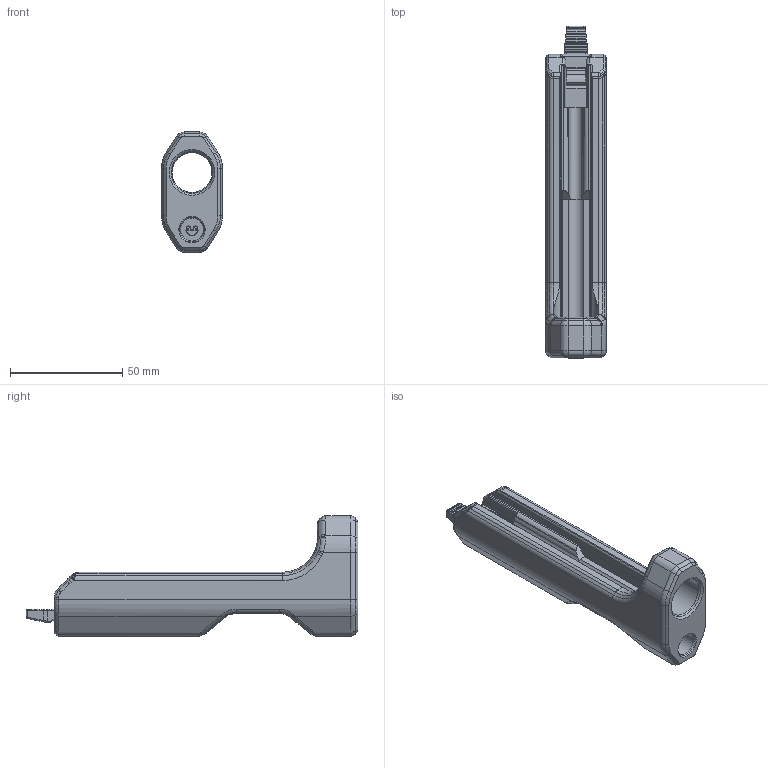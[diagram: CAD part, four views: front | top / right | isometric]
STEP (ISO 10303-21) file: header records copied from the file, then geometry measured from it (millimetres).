
FILE_DESCRIPTION(/* description */ (''),/* implementation_level */ '2;1');
FILE_NAME(/* name */ '10mm Spike Mount.step',/* time_stamp */ '2021-09-22T07:34:55-04:00',/* author */ (''),/* organization */ (''),/* preprocessor_version */ 'ST-DEVELOPER v18.1',/* originating_system */ 'Autodesk Translation Framework v10.10.0.1391',/* authorisation */ '');
FILE_SCHEMA (('AUTOMOTIVE_DESIGN { 1 0 10303 214 3 1 1 }'));
Length unit declared in the file: millimetre
Products named in the file (1): 10mm Spike
Bounding box: 27 x 147.6 x 53.45 mm (x, y, z)
Volume: 68152.1 mm3; surface area: 22846.5 mm2
Topology: 1 solids, 1 shells, 507 faces, 1249 edges, 740 vertices
Faces by surface type: cylinder 161, bspline 152, plane 112, torus 51, cone 25, sphere 6
Full cylindrical faces by diameter (mm): 10.2 x1, 17.8 x1
Entity records: 18304 total; most frequent: CARTESIAN_POINT 7053, ORIENTED_EDGE 2490, DIRECTION 2142, EDGE_CURVE 1245, AXIS2_PLACEMENT_3D 827, VERTEX_POINT 740, EDGE_LOOP 513, FACE_OUTER_BOUND 507
